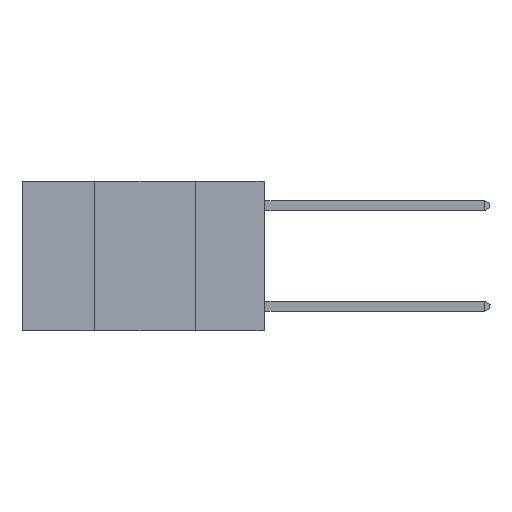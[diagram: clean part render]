
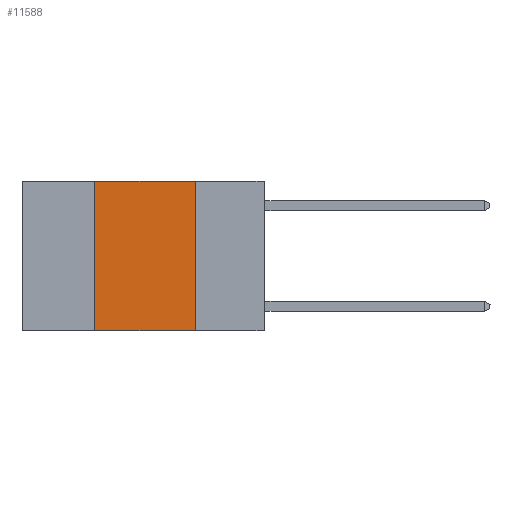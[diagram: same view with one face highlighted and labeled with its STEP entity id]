
A CAD part, left-side view. The second image highlights one B-rep face of the part: STEP entity #11588.
In plain terms, the highlighted planar face has unit normal (-1, 0, 0).
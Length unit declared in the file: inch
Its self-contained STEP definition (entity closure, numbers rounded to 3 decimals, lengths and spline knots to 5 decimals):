
#121 = ORIENTED_EDGE ( 'NONE', *, *, #5388, .F. ) ;
#181 = EDGE_CURVE ( 'NONE', #7683, #13846, #12824, .T. ) ;
#213 = VECTOR ( 'NONE', #20740, 39.37008 ) ;
#1199 = ORIENTED_EDGE ( 'NONE', *, *, #20611, .T. ) ;
#1465 = CARTESIAN_POINT ( 'NONE',  ( 0., 0.6, -0.37 ) ) ;
#2537 = VECTOR ( 'NONE', #20350, 39.37008 ) ;
#2810 = DIRECTION ( 'NONE',  ( 0., -1., 0. ) ) ;
#3117 = VECTOR ( 'NONE', #2810, 39.37008 ) ;
#5263 = CARTESIAN_POINT ( 'NONE',  ( 0., 0.42, 0. ) ) ;
#5388 = EDGE_CURVE ( 'NONE', #15930, #7068, #15649, .T. ) ;
#7068 = VERTEX_POINT ( 'NONE', #15344 ) ;
#7683 = VERTEX_POINT ( 'NONE', #22832 ) ;
#8464 = CARTESIAN_POINT ( 'NONE',  ( 0., 0.6, 0. ) ) ;
#8621 = CARTESIAN_POINT ( 'NONE',  ( 0., 0.6, 0. ) ) ;
#11224 = ORIENTED_EDGE ( 'NONE', *, *, #181, .F. ) ;
#11588 = ADVANCED_FACE ( 'NONE', ( #22098 ), #21937, .F. ) ;
#12334 = DIRECTION ( 'NONE',  ( 0., 0., -1. ) ) ;
#12824 = LINE ( 'NONE', #20321, #2537 ) ;
#13761 = EDGE_LOOP ( 'NONE', ( #11224, #21473, #121, #1199 ) ) ;
#13846 = VERTEX_POINT ( 'NONE', #15147 ) ;
#15147 = CARTESIAN_POINT ( 'NONE',  ( 0., 0.17, -0.37 ) ) ;
#15344 = CARTESIAN_POINT ( 'NONE',  ( 0., 0.42, 0. ) ) ;
#15649 = LINE ( 'NONE', #5263, #213 ) ;
#15879 = LINE ( 'NONE', #1465, #17714 ) ;
#15930 = VERTEX_POINT ( 'NONE', #22822 ) ;
#17366 = LINE ( 'NONE', #8621, #3117 ) ;
#17714 = VECTOR ( 'NONE', #22761, 39.37008 ) ;
#20321 = CARTESIAN_POINT ( 'NONE',  ( 0., 0.17, 0. ) ) ;
#20350 = DIRECTION ( 'NONE',  ( 0., 0., -1. ) ) ;
#20611 = EDGE_CURVE ( 'NONE', #15930, #13846, #15879, .T. ) ;
#20740 = DIRECTION ( 'NONE',  ( 0., 0., 1. ) ) ;
#21473 = ORIENTED_EDGE ( 'NONE', *, *, #22307, .F. ) ;
#21937 = PLANE ( 'NONE',  #22120 ) ;
#22098 = FACE_OUTER_BOUND ( 'NONE', #13761, .T. ) ;
#22120 = AXIS2_PLACEMENT_3D ( 'NONE', #8464, #23866, #12334 ) ;
#22307 = EDGE_CURVE ( 'NONE', #7068, #7683, #17366, .T. ) ;
#22761 = DIRECTION ( 'NONE',  ( 0., -1., 0. ) ) ;
#22822 = CARTESIAN_POINT ( 'NONE',  ( 0., 0.42, -0.37 ) ) ;
#22832 = CARTESIAN_POINT ( 'NONE',  ( 0., 0.17, 0. ) ) ;
#23866 = DIRECTION ( 'NONE',  ( 1., 0., 0. ) ) ;
